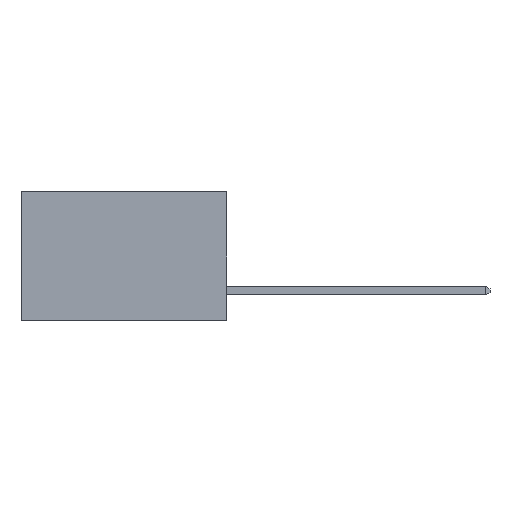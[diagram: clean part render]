
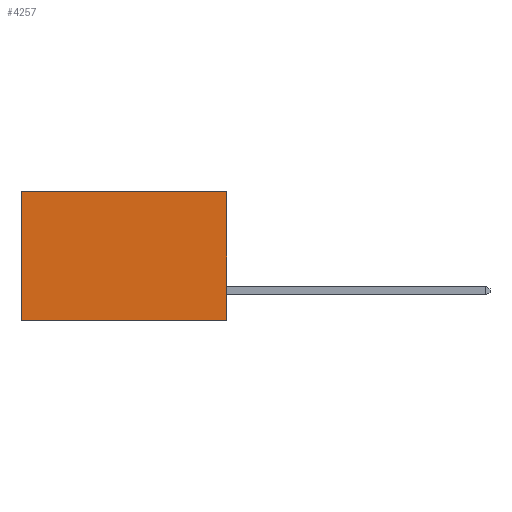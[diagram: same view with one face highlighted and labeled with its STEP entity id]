
A CAD part, left-side view. The second image highlights one B-rep face of the part: STEP entity #4257.
In plain terms, the highlighted planar face has unit normal (-1, 0, 0).
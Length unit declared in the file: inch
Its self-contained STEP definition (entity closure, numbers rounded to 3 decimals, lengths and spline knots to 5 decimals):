
#542 = CARTESIAN_POINT ( 'NONE',  ( 0.277, 0.59, -0.37 ) ) ;
#691 = LINE ( 'NONE', #6230, #8938 ) ;
#1258 = EDGE_CURVE ( 'NONE', #2670, #2231, #1803, .T. ) ;
#1803 = LINE ( 'NONE', #6551, #7255 ) ;
#2175 = AXIS2_PLACEMENT_3D ( 'NONE', #7802, #7792, #7756 ) ;
#2231 = VERTEX_POINT ( 'NONE', #542 ) ;
#2670 = VERTEX_POINT ( 'NONE', #4841 ) ;
#4257 = ADVANCED_FACE ( 'NONE', ( #6631 ), #7885, .F. ) ;
#4434 = EDGE_CURVE ( 'NONE', #10592, #2231, #691, .T. ) ;
#4482 = CARTESIAN_POINT ( 'NONE',  ( 0.277, 0., -0.37 ) ) ;
#4841 = CARTESIAN_POINT ( 'NONE',  ( 0.277, 0., -0.37 ) ) ;
#5076 = EDGE_CURVE ( 'NONE', #11401, #10592, #8750, .T. ) ;
#5908 = VECTOR ( 'NONE', #11949, 39.37008 ) ;
#6197 = DIRECTION ( 'NONE',  ( 0., 0., -1. ) ) ;
#6230 = CARTESIAN_POINT ( 'NONE',  ( 0.277, 0.59, -0.37 ) ) ;
#6551 = CARTESIAN_POINT ( 'NONE',  ( 0.277, 0., -0.37 ) ) ;
#6631 = FACE_OUTER_BOUND ( 'NONE', #11554, .T. ) ;
#6656 = DIRECTION ( 'NONE',  ( 0., 1., 0. ) ) ;
#6728 = DIRECTION ( 'NONE',  ( 0., 0., -1. ) ) ;
#7168 = VECTOR ( 'NONE', #6728, 39.37008 ) ;
#7255 = VECTOR ( 'NONE', #6656, 39.37008 ) ;
#7756 = DIRECTION ( 'NONE',  ( 0., 0., -1. ) ) ;
#7792 = DIRECTION ( 'NONE',  ( 1., 0., 0. ) ) ;
#7802 = CARTESIAN_POINT ( 'NONE',  ( 0.277, 0., -0.37 ) ) ;
#7885 = PLANE ( 'NONE',  #2175 ) ;
#8750 = LINE ( 'NONE', #12224, #5908 ) ;
#8938 = VECTOR ( 'NONE', #6197, 39.37008 ) ;
#9358 = CARTESIAN_POINT ( 'NONE',  ( 0.277, 0.59, 0. ) ) ;
#9847 = ORIENTED_EDGE ( 'NONE', *, *, #4434, .T. ) ;
#9912 = LINE ( 'NONE', #4482, #7168 ) ;
#10047 = ORIENTED_EDGE ( 'NONE', *, *, #1258, .F. ) ;
#10131 = ORIENTED_EDGE ( 'NONE', *, *, #11580, .F. ) ;
#10592 = VERTEX_POINT ( 'NONE', #9358 ) ;
#10997 = ORIENTED_EDGE ( 'NONE', *, *, #5076, .T. ) ;
#11401 = VERTEX_POINT ( 'NONE', #12714 ) ;
#11554 = EDGE_LOOP ( 'NONE', ( #9847, #10047, #10131, #10997 ) ) ;
#11580 = EDGE_CURVE ( 'NONE', #11401, #2670, #9912, .T. ) ;
#11949 = DIRECTION ( 'NONE',  ( 0., 1., 0. ) ) ;
#12224 = CARTESIAN_POINT ( 'NONE',  ( 0.277, 0., 0. ) ) ;
#12714 = CARTESIAN_POINT ( 'NONE',  ( 0.277, 0., 0. ) ) ;
